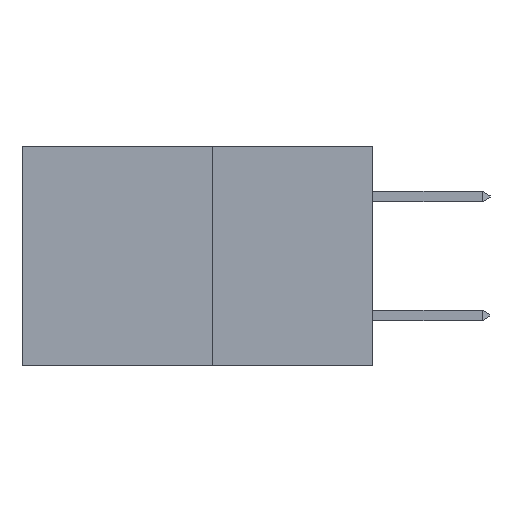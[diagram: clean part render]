
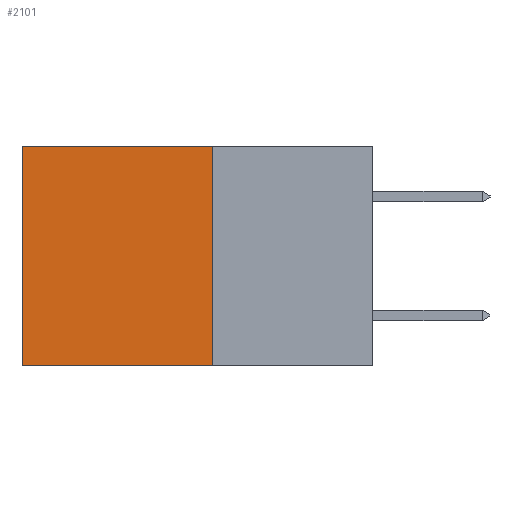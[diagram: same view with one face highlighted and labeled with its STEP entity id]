
A CAD part, left-side view. The second image highlights one B-rep face of the part: STEP entity #2101.
In plain terms, the highlighted planar face has unit normal (-1, 0, 0).
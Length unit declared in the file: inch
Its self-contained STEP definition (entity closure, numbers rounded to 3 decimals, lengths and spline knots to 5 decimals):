
#199 = VECTOR ( 'NONE', #8197, 39.37008 ) ;
#1567 = EDGE_CURVE ( 'NONE', #7949, #13909, #5838, .T. ) ;
#1852 = CARTESIAN_POINT ( 'NONE',  ( 0.277, 0.27, 0. ) ) ;
#2101 = ADVANCED_FACE ( 'NONE', ( #6469 ), #8118, .F. ) ;
#2467 = CARTESIAN_POINT ( 'NONE',  ( 0.277, 0.27, -0.37 ) ) ;
#2483 = VECTOR ( 'NONE', #9966, 39.37008 ) ;
#3003 = DIRECTION ( 'NONE',  ( 1., 0., 0. ) ) ;
#4990 = VERTEX_POINT ( 'NONE', #2467 ) ;
#5551 = ORIENTED_EDGE ( 'NONE', *, *, #1567, .T. ) ;
#5838 = LINE ( 'NONE', #1852, #2483 ) ;
#6085 = CARTESIAN_POINT ( 'NONE',  ( 0.277, 0.59, 0. ) ) ;
#6152 = VECTOR ( 'NONE', #8415, 39.37008 ) ;
#6469 = FACE_OUTER_BOUND ( 'NONE', #12550, .T. ) ;
#6521 = ORIENTED_EDGE ( 'NONE', *, *, #16230, .F. ) ;
#7000 = CARTESIAN_POINT ( 'NONE',  ( 0.277, 0.27, -0.37 ) ) ;
#7014 = EDGE_CURVE ( 'NONE', #13909, #12922, #14984, .T. ) ;
#7423 = ORIENTED_EDGE ( 'NONE', *, *, #12434, .F. ) ;
#7949 = VERTEX_POINT ( 'NONE', #17411 ) ;
#8022 = CARTESIAN_POINT ( 'NONE',  ( 0.277, 0.27, -0.37 ) ) ;
#8118 = PLANE ( 'NONE',  #9664 ) ;
#8197 = DIRECTION ( 'NONE',  ( 0., 0., -1. ) ) ;
#8415 = DIRECTION ( 'NONE',  ( 0., 0., -1. ) ) ;
#9264 = DIRECTION ( 'NONE',  ( 0., 0., -1. ) ) ;
#9664 = AXIS2_PLACEMENT_3D ( 'NONE', #14722, #3003, #9264 ) ;
#9966 = DIRECTION ( 'NONE',  ( 0., 1., 0. ) ) ;
#10092 = VECTOR ( 'NONE', #12372, 39.37008 ) ;
#10881 = CARTESIAN_POINT ( 'NONE',  ( 0.277, 0.59, -0.37 ) ) ;
#12372 = DIRECTION ( 'NONE',  ( 0., 1., 0. ) ) ;
#12434 = EDGE_CURVE ( 'NONE', #7949, #4990, #17260, .T. ) ;
#12550 = EDGE_LOOP ( 'NONE', ( #16095, #6521, #7423, #5551 ) ) ;
#12922 = VERTEX_POINT ( 'NONE', #10881 ) ;
#13884 = LINE ( 'NONE', #8022, #10092 ) ;
#13909 = VERTEX_POINT ( 'NONE', #6085 ) ;
#14722 = CARTESIAN_POINT ( 'NONE',  ( 0.277, 0.27, -0.37 ) ) ;
#14984 = LINE ( 'NONE', #16706, #199 ) ;
#16095 = ORIENTED_EDGE ( 'NONE', *, *, #7014, .T. ) ;
#16230 = EDGE_CURVE ( 'NONE', #4990, #12922, #13884, .T. ) ;
#16706 = CARTESIAN_POINT ( 'NONE',  ( 0.277, 0.59, -0.37 ) ) ;
#17260 = LINE ( 'NONE', #7000, #6152 ) ;
#17411 = CARTESIAN_POINT ( 'NONE',  ( 0.277, 0.27, 0. ) ) ;
